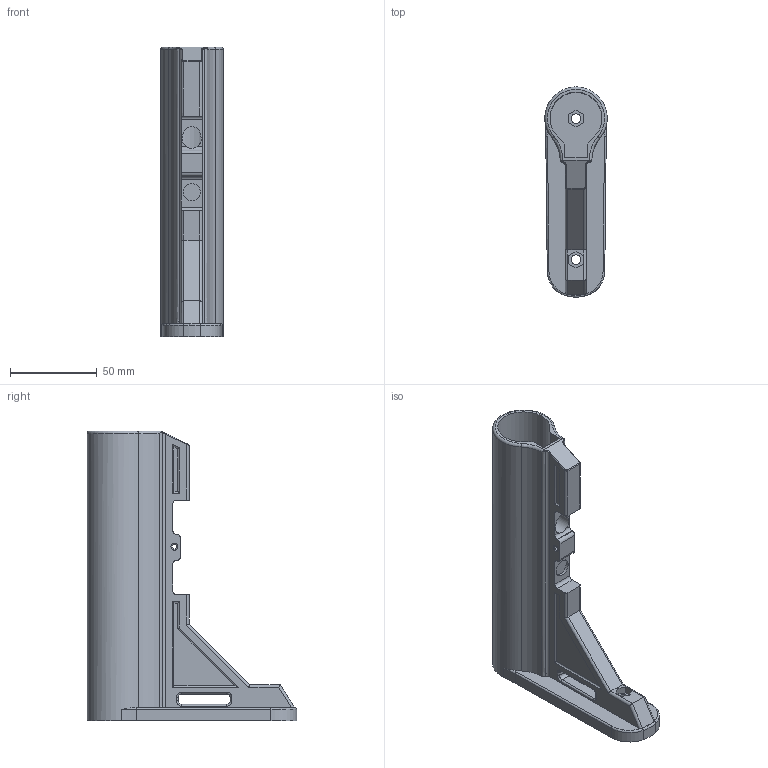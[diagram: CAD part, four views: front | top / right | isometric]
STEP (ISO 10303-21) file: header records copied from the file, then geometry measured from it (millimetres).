
FILE_DESCRIPTION(/* description */ (''),/* implementation_level */ '2;1');
FILE_NAME(/* name */ 'Custom Stock Body.step',/* time_stamp */ '2022-05-27T20:29:53-05:00',/* author */ (''),/* organization */ (''),/* preprocessor_version */ 'ST-DEVELOPER v19',/* originating_system */ 'Autodesk Translation Framework v11.7.0.108',/* authorisation */ '');
FILE_SCHEMA (('AUTOMOTIVE_DESIGN { 1 0 10303 214 3 1 1 }'));
Length unit declared in the file: millimetre
Products named in the file (1): Custom Stock
Bounding box: 35.98 x 120.93 x 167.07 mm (x, y, z)
Volume: 122215.2 mm3; surface area: 55474.3 mm2
Topology: 1 solids, 1 shells, 149 faces, 382 edges, 243 vertices
Faces by surface type: cylinder 70, plane 53, torus 18, bspline 8
Full cylindrical faces by diameter (mm): 3 x1, 5.5 x2, 10 x1
Entity records: 4910 total; most frequent: CARTESIAN_POINT 1167, DIRECTION 791, ORIENTED_EDGE 764, EDGE_CURVE 382, AXIS2_PLACEMENT_3D 293, VERTEX_POINT 243, LINE 205, VECTOR 205
